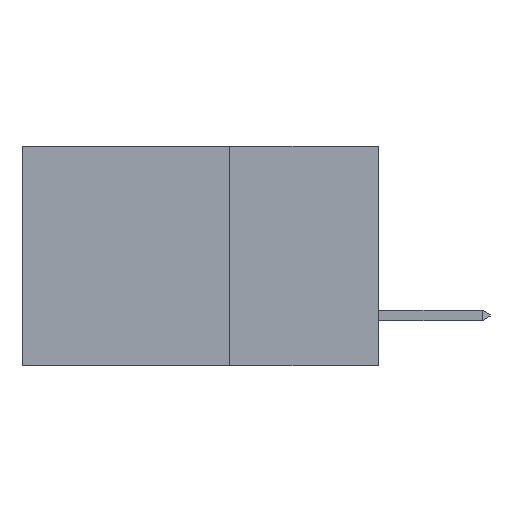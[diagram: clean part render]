
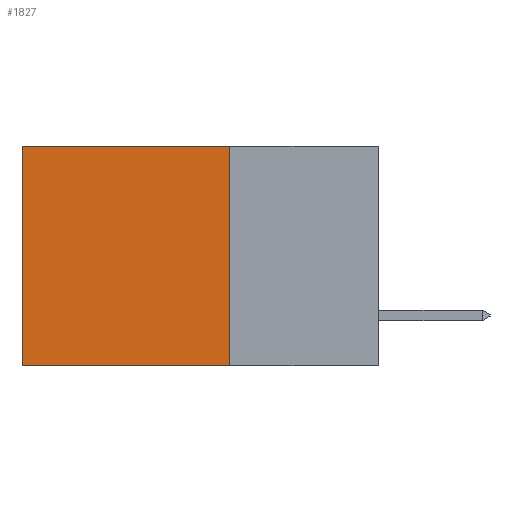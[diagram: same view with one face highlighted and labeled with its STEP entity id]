
A CAD part, left-side view. The second image highlights one B-rep face of the part: STEP entity #1827.
In plain terms, the highlighted planar face has unit normal (-1, 0, 0).
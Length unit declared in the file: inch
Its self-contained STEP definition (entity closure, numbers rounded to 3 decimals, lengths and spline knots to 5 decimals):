
#132 = VECTOR ( 'NONE', #10622, 39.37008 ) ;
#609 = CARTESIAN_POINT ( 'NONE',  ( 0.298, 0.25, 0. ) ) ;
#823 = EDGE_CURVE ( 'NONE', #1982, #1336, #9124, .T. ) ;
#1071 = CARTESIAN_POINT ( 'NONE',  ( 0.298, 0.25, -0.37 ) ) ;
#1219 = VECTOR ( 'NONE', #3687, 39.37008 ) ;
#1336 = VERTEX_POINT ( 'NONE', #1403 ) ;
#1403 = CARTESIAN_POINT ( 'NONE',  ( 0.298, 0.6, -0.37 ) ) ;
#1576 = LINE ( 'NONE', #8891, #1219 ) ;
#1827 = ADVANCED_FACE ( 'NONE', ( #6769 ), #3017, .F. ) ;
#1982 = VERTEX_POINT ( 'NONE', #1071 ) ;
#2128 = VERTEX_POINT ( 'NONE', #4109 ) ;
#2251 = EDGE_CURVE ( 'NONE', #2128, #1336, #1576, .T. ) ;
#2613 = DIRECTION ( 'NONE',  ( 0., 1., 0. ) ) ;
#2911 = ORIENTED_EDGE ( 'NONE', *, *, #2251, .T. ) ;
#2976 = ORIENTED_EDGE ( 'NONE', *, *, #823, .F. ) ;
#3000 = LINE ( 'NONE', #5750, #132 ) ;
#3017 = PLANE ( 'NONE',  #4552 ) ;
#3058 = ORIENTED_EDGE ( 'NONE', *, *, #12341, .F. ) ;
#3071 = ORIENTED_EDGE ( 'NONE', *, *, #9783, .T. ) ;
#3687 = DIRECTION ( 'NONE',  ( 0., 0., -1. ) ) ;
#4109 = CARTESIAN_POINT ( 'NONE',  ( 0.298, 0.6, 0. ) ) ;
#4552 = AXIS2_PLACEMENT_3D ( 'NONE', #9825, #9784, #11022 ) ;
#5750 = CARTESIAN_POINT ( 'NONE',  ( 0.298, 0.25, 0. ) ) ;
#5885 = DIRECTION ( 'NONE',  ( 0., 1., 0. ) ) ;
#6478 = VECTOR ( 'NONE', #2613, 39.37008 ) ;
#6769 = FACE_OUTER_BOUND ( 'NONE', #9861, .T. ) ;
#7304 = VERTEX_POINT ( 'NONE', #12938 ) ;
#7975 = LINE ( 'NONE', #609, #9899 ) ;
#8891 = CARTESIAN_POINT ( 'NONE',  ( 0.298, 0.6, 0. ) ) ;
#8920 = CARTESIAN_POINT ( 'NONE',  ( 0.298, 0.25, -0.37 ) ) ;
#9124 = LINE ( 'NONE', #8920, #6478 ) ;
#9783 = EDGE_CURVE ( 'NONE', #7304, #2128, #7975, .T. ) ;
#9784 = DIRECTION ( 'NONE',  ( 1., 0., 0. ) ) ;
#9825 = CARTESIAN_POINT ( 'NONE',  ( 0.298, 0.25, 0. ) ) ;
#9861 = EDGE_LOOP ( 'NONE', ( #2911, #2976, #3058, #3071 ) ) ;
#9899 = VECTOR ( 'NONE', #5885, 39.37008 ) ;
#10622 = DIRECTION ( 'NONE',  ( 0., 0., -1. ) ) ;
#11022 = DIRECTION ( 'NONE',  ( 0., 0., -1. ) ) ;
#12341 = EDGE_CURVE ( 'NONE', #7304, #1982, #3000, .T. ) ;
#12938 = CARTESIAN_POINT ( 'NONE',  ( 0.298, 0.25, 0. ) ) ;
